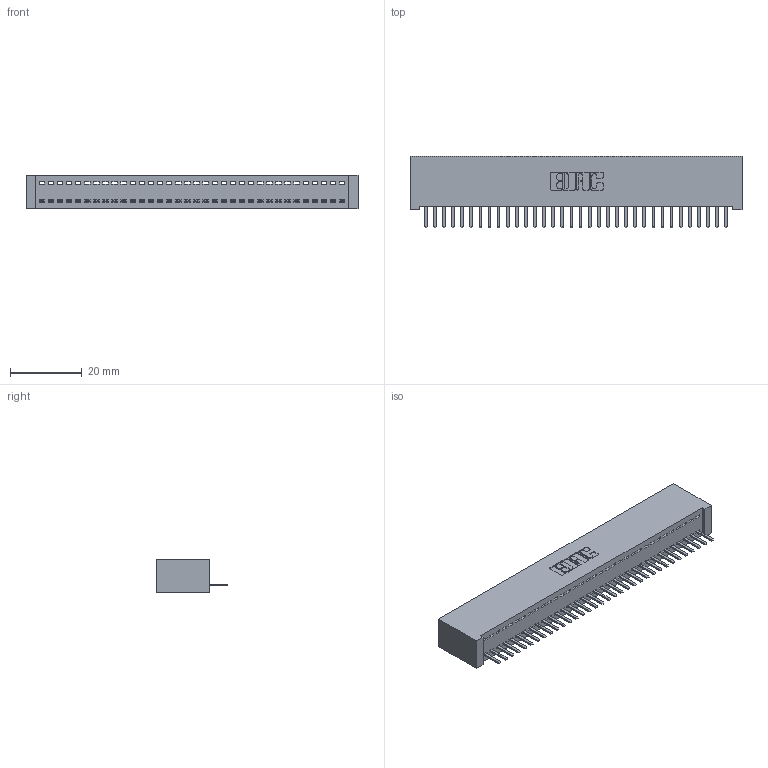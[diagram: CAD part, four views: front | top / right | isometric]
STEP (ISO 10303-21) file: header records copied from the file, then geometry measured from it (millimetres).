
FILE_DESCRIPTION (( 'STEP AP203' ), '1' );
FILE_NAME ('342-034-520-101.STEP', '2018-08-11T18:07:26', ( '' ), ( '' ), 'SwSTEP 2.0', 'SolidWorks 2016', '' );
FILE_SCHEMA (( 'CONFIG_CONTROL_DESIGN' ));
Length unit declared in the file: inch
Products named in the file (3): 345-292-001_345-293-120; 342-034-520-101; 342 Part_Lugless
Assembly tree (35 placements, depth 2):
  342-034-520-101
    342 Part_Lugless
    345-292-001_345-293-120  x34
Bounding box: 92.61 x 20.02 x 9.4 mm (x, y, z)
Volume: 8401.6 mm3; surface area: 12198.5 mm2
Topology: 35 solids, 35 shells, 2210 faces, 6531 edges, 4262 vertices
Faces by surface type: plane 1558, cylinder 652
Entity records: 21525 total; most frequent: CARTESIAN_POINT 3732, ORIENTED_EDGE 3690, DIRECTION 3145, EDGE_CURVE 1845, VECTOR 1721, LINE 1721, VERTEX_POINT 1226, AXIS2_PLACEMENT_3D 712
